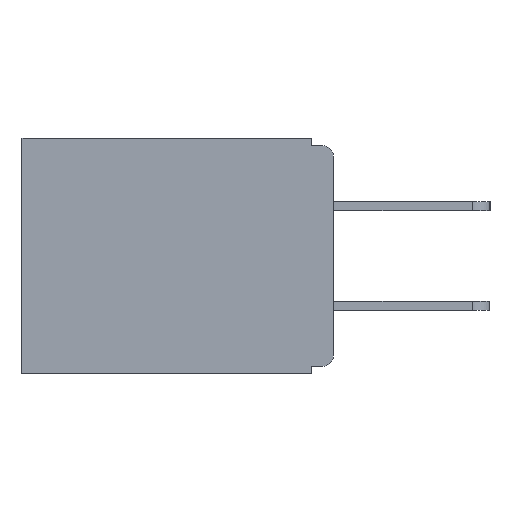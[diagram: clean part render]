
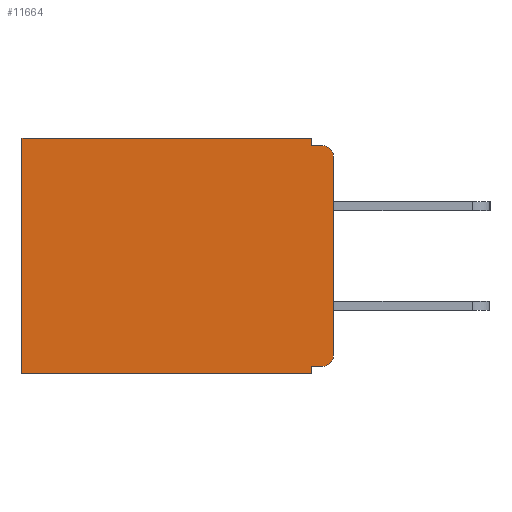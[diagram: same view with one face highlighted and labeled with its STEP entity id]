
A CAD part, left-side view. The second image highlights one B-rep face of the part: STEP entity #11664.
In plain terms, the highlighted planar face has unit normal (-1, 0, 0).
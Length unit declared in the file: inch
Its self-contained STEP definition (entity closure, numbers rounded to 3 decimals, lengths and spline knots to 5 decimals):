
#236 = LINE ( 'NONE', #10398, #13838 ) ;
#366 = ORIENTED_EDGE ( 'NONE', *, *, #12438, .F. ) ;
#473 = DIRECTION ( 'NONE',  ( 1., 0., 0. ) ) ;
#1504 = VECTOR ( 'NONE', #17851, 39.37008 ) ;
#1561 = DIRECTION ( 'NONE',  ( 0., 0., -1. ) ) ;
#2020 = CARTESIAN_POINT ( 'NONE',  ( 0.3, 0.437, -0.33 ) ) ;
#2309 = VERTEX_POINT ( 'NONE', #10983 ) ;
#2406 = EDGE_CURVE ( 'NONE', #2309, #14871, #236, .T. ) ;
#2521 = VECTOR ( 'NONE', #14331, 39.37008 ) ;
#2742 = ORIENTED_EDGE ( 'NONE', *, *, #13466, .F. ) ;
#3130 = ORIENTED_EDGE ( 'NONE', *, *, #11159, .T. ) ;
#3392 = ORIENTED_EDGE ( 'NONE', *, *, #8955, .F. ) ;
#3724 = LINE ( 'NONE', #18219, #13053 ) ;
#3980 = VECTOR ( 'NONE', #14682, 39.37008 ) ;
#4665 = VERTEX_POINT ( 'NONE', #7872 ) ;
#4745 = VERTEX_POINT ( 'NONE', #16162 ) ;
#4833 = DIRECTION ( 'NONE',  ( 0., 0., -1. ) ) ;
#5056 = LINE ( 'NONE', #13027, #3980 ) ;
#5632 = VERTEX_POINT ( 'NONE', #6673 ) ;
#5711 = CARTESIAN_POINT ( 'NONE',  ( 0.3, 0., 0. ) ) ;
#5864 = CARTESIAN_POINT ( 'NONE',  ( 0.3, 0., -0.33 ) ) ;
#6207 = DIRECTION ( 'NONE',  ( 0., 0., -1. ) ) ;
#6272 = DIRECTION ( 'NONE',  ( -1., 0., 0. ) ) ;
#6411 = EDGE_CURVE ( 'NONE', #5632, #14871, #15264, .T. ) ;
#6673 = CARTESIAN_POINT ( 'NONE',  ( 0.3, 0.015, -0.32 ) ) ;
#7872 = CARTESIAN_POINT ( 'NONE',  ( 0.3, 0.031, -0.01 ) ) ;
#8092 = CARTESIAN_POINT ( 'NONE',  ( 0.3, 0.031, -0.33 ) ) ;
#8955 = EDGE_CURVE ( 'NONE', #14958, #16767, #10618, .T. ) ;
#9564 = DIRECTION ( 'NONE',  ( 0., -1., 0. ) ) ;
#9983 = EDGE_CURVE ( 'NONE', #11375, #20684, #11933, .T. ) ;
#9993 = CARTESIAN_POINT ( 'NONE',  ( 0.3, 0.031, -0.33 ) ) ;
#10001 = VECTOR ( 'NONE', #4833, 39.37008 ) ;
#10224 = ORIENTED_EDGE ( 'NONE', *, *, #21529, .F. ) ;
#10240 = CIRCLE ( 'NONE', #17279, 0.015 ) ;
#10398 = CARTESIAN_POINT ( 'NONE',  ( 0.3, 0., -0.33 ) ) ;
#10470 = LINE ( 'NONE', #5711, #1504 ) ;
#10618 = LINE ( 'NONE', #8092, #16253 ) ;
#10851 = EDGE_LOOP ( 'NONE', ( #18472, #3130, #17967, #366, #17393, #17908, #10224, #3392, #2742, #14607 ) ) ;
#10983 = CARTESIAN_POINT ( 'NONE',  ( 0.3, 0., -0.025 ) ) ;
#11159 = EDGE_CURVE ( 'NONE', #2309, #16835, #10240, .T. ) ;
#11375 = VERTEX_POINT ( 'NONE', #20538 ) ;
#11664 = ADVANCED_FACE ( 'NONE', ( #12610 ), #17994, .F. ) ;
#11886 = CARTESIAN_POINT ( 'NONE',  ( 0.3, 0.015, -0.01 ) ) ;
#11933 = LINE ( 'NONE', #2020, #2521 ) ;
#12438 = EDGE_CURVE ( 'NONE', #4745, #4665, #19054, .T. ) ;
#12610 = FACE_OUTER_BOUND ( 'NONE', #10851, .T. ) ;
#12926 = DIRECTION ( 'NONE',  ( 0., 0., -1. ) ) ;
#13027 = CARTESIAN_POINT ( 'NONE',  ( 0.3, 0., -0.33 ) ) ;
#13053 = VECTOR ( 'NONE', #9564, 39.37008 ) ;
#13466 = EDGE_CURVE ( 'NONE', #5632, #14958, #16381, .T. ) ;
#13838 = VECTOR ( 'NONE', #18225, 39.37008 ) ;
#14118 = AXIS2_PLACEMENT_3D ( 'NONE', #5864, #473, #12926 ) ;
#14331 = DIRECTION ( 'NONE',  ( 0., 0., -1. ) ) ;
#14359 = EDGE_CURVE ( 'NONE', #4745, #11375, #10470, .T. ) ;
#14607 = ORIENTED_EDGE ( 'NONE', *, *, #6411, .T. ) ;
#14682 = DIRECTION ( 'NONE',  ( 0., 1., 0. ) ) ;
#14871 = VERTEX_POINT ( 'NONE', #22349 ) ;
#14958 = VERTEX_POINT ( 'NONE', #15898 ) ;
#15264 = CIRCLE ( 'NONE', #20628, 0.015 ) ;
#15842 = VECTOR ( 'NONE', #16372, 39.37008 ) ;
#15898 = CARTESIAN_POINT ( 'NONE',  ( 0.3, 0.031, -0.32 ) ) ;
#16162 = CARTESIAN_POINT ( 'NONE',  ( 0.3, 0.031, 0. ) ) ;
#16253 = VECTOR ( 'NONE', #6207, 39.37008 ) ;
#16372 = DIRECTION ( 'NONE',  ( 0., 1., 0. ) ) ;
#16381 = LINE ( 'NONE', #17998, #15842 ) ;
#16699 = CARTESIAN_POINT ( 'NONE',  ( 0.3, 0.015, -0.025 ) ) ;
#16767 = VERTEX_POINT ( 'NONE', #9993 ) ;
#16835 = VERTEX_POINT ( 'NONE', #11886 ) ;
#17023 = CARTESIAN_POINT ( 'NONE',  ( 0.3, 0.031, 0. ) ) ;
#17279 = AXIS2_PLACEMENT_3D ( 'NONE', #16699, #6272, #18356 ) ;
#17393 = ORIENTED_EDGE ( 'NONE', *, *, #14359, .T. ) ;
#17851 = DIRECTION ( 'NONE',  ( 0., 1., 0. ) ) ;
#17908 = ORIENTED_EDGE ( 'NONE', *, *, #9983, .T. ) ;
#17967 = ORIENTED_EDGE ( 'NONE', *, *, #20334, .F. ) ;
#17994 = PLANE ( 'NONE',  #14118 ) ;
#17998 = CARTESIAN_POINT ( 'NONE',  ( 0.3, 0., -0.32 ) ) ;
#18219 = CARTESIAN_POINT ( 'NONE',  ( 0.3, 0., -0.01 ) ) ;
#18225 = DIRECTION ( 'NONE',  ( 0., 0., -1. ) ) ;
#18356 = DIRECTION ( 'NONE',  ( 0., 0., -1. ) ) ;
#18472 = ORIENTED_EDGE ( 'NONE', *, *, #2406, .F. ) ;
#19054 = LINE ( 'NONE', #17023, #10001 ) ;
#19111 = CARTESIAN_POINT ( 'NONE',  ( 0.3, 0.015, -0.305 ) ) ;
#20334 = EDGE_CURVE ( 'NONE', #4665, #16835, #3724, .T. ) ;
#20538 = CARTESIAN_POINT ( 'NONE',  ( 0.3, 0.437, 0. ) ) ;
#20628 = AXIS2_PLACEMENT_3D ( 'NONE', #19111, #21121, #1561 ) ;
#20684 = VERTEX_POINT ( 'NONE', #20891 ) ;
#20891 = CARTESIAN_POINT ( 'NONE',  ( 0.3, 0.437, -0.33 ) ) ;
#21121 = DIRECTION ( 'NONE',  ( -1., 0., 0. ) ) ;
#21529 = EDGE_CURVE ( 'NONE', #16767, #20684, #5056, .T. ) ;
#22349 = CARTESIAN_POINT ( 'NONE',  ( 0.3, 0., -0.305 ) ) ;
